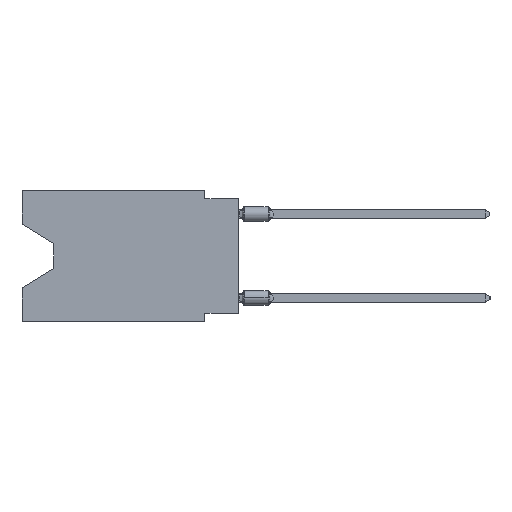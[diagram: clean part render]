
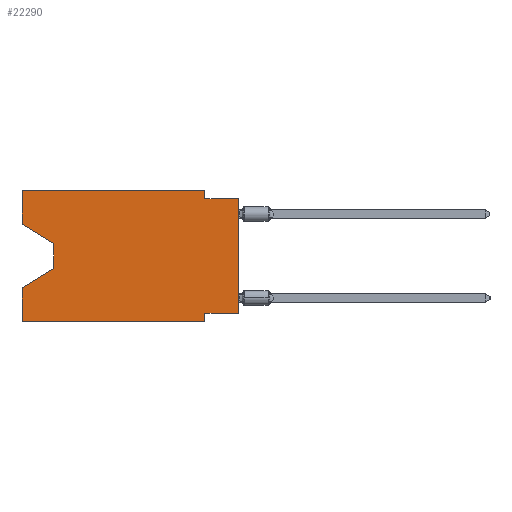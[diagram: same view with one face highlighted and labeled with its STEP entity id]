
A CAD part, left-side view. The second image highlights one B-rep face of the part: STEP entity #22290.
In plain terms, the highlighted planar face has unit normal (-1, 0, 0).
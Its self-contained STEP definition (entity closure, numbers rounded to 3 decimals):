
#914 = ORIENTED_EDGE ( 'NONE', *, *, #37291, .T. ) ;
#1246 = VECTOR ( 'NONE', #50071, 1000. ) ;
#2125 = FACE_OUTER_BOUND ( 'NONE', #40277, .T. ) ;
#2347 = LINE ( 'NONE', #66242, #57676 ) ;
#2634 = ORIENTED_EDGE ( 'NONE', *, *, #29283, .T. ) ;
#2832 = CARTESIAN_POINT ( 'NONE',  ( 0., 16.383, 0. ) ) ;
#3157 = CARTESIAN_POINT ( 'NONE',  ( 0., 0., -9.271 ) ) ;
#3553 = CARTESIAN_POINT ( 'NONE',  ( 0., 13.97, -5.893 ) ) ;
#3563 = ORIENTED_EDGE ( 'NONE', *, *, #9586, .F. ) ;
#4128 = VERTEX_POINT ( 'NONE', #50631 ) ;
#4748 = CARTESIAN_POINT ( 'NONE',  ( 0., 16.383, 0. ) ) ;
#4784 = ORIENTED_EDGE ( 'NONE', *, *, #48665, .F. ) ;
#5268 = LINE ( 'NONE', #67221, #38157 ) ;
#5447 = VERTEX_POINT ( 'NONE', #4748 ) ;
#6087 = CARTESIAN_POINT ( 'NONE',  ( 0., 2.54, 0. ) ) ;
#6131 = EDGE_CURVE ( 'NONE', #46796, #10814, #5268, .T. ) ;
#6180 = CARTESIAN_POINT ( 'NONE',  ( 0., 0., 0. ) ) ;
#6222 = VECTOR ( 'NONE', #42809, 1000. ) ;
#8156 = VERTEX_POINT ( 'NONE', #3553 ) ;
#9586 = EDGE_CURVE ( 'NONE', #55805, #35050, #18229, .T. ) ;
#9799 = EDGE_CURVE ( 'NONE', #63018, #8156, #32179, .T. ) ;
#10131 = ORIENTED_EDGE ( 'NONE', *, *, #9799, .T. ) ;
#10814 = VERTEX_POINT ( 'NONE', #50067 ) ;
#11669 = DIRECTION ( 'NONE',  ( 0., 0., 1. ) ) ;
#11736 = EDGE_CURVE ( 'NONE', #55805, #40909, #49175, .T. ) ;
#12637 = DIRECTION ( 'NONE',  ( 0., 0.855, -0.519 ) ) ;
#12690 = LINE ( 'NONE', #6180, #13925 ) ;
#12749 = VECTOR ( 'NONE', #59636, 1000. ) ;
#12761 = DIRECTION ( 'NONE',  ( 0., 0., -1. ) ) ;
#13824 = CARTESIAN_POINT ( 'NONE',  ( 0., 2.54, -9.906 ) ) ;
#13925 = VECTOR ( 'NONE', #11669, 1000. ) ;
#14439 = LINE ( 'NONE', #3157, #66631 ) ;
#14901 = DIRECTION ( 'NONE',  ( 0., 0., -1. ) ) ;
#15201 = DIRECTION ( 'NONE',  ( 0., -1., 0. ) ) ;
#16277 = VECTOR ( 'NONE', #25851, 1000. ) ;
#16648 = VERTEX_POINT ( 'NONE', #6087 ) ;
#17087 = CARTESIAN_POINT ( 'NONE',  ( 0., 16.383, 0. ) ) ;
#17767 = DIRECTION ( 'NONE',  ( 0., 0., 1. ) ) ;
#18229 = LINE ( 'NONE', #43891, #12749 ) ;
#18454 = ORIENTED_EDGE ( 'NONE', *, *, #25771, .F. ) ;
#18570 = DIRECTION ( 'NONE',  ( 0., 1., 0. ) ) ;
#21755 = LINE ( 'NONE', #53243, #16277 ) ;
#22000 = DIRECTION ( 'NONE',  ( 1., 0., 0. ) ) ;
#22219 = LINE ( 'NONE', #17087, #60879 ) ;
#22290 = ADVANCED_FACE ( 'NONE', ( #2125 ), #37730, .F. ) ;
#23151 = CARTESIAN_POINT ( 'NONE',  ( 0., 16.383, -9.906 ) ) ;
#25771 = EDGE_CURVE ( 'NONE', #4128, #40909, #51959, .T. ) ;
#25851 = DIRECTION ( 'NONE',  ( 0., -0.855, -0.519 ) ) ;
#26145 = ORIENTED_EDGE ( 'NONE', *, *, #6131, .F. ) ;
#26645 = VERTEX_POINT ( 'NONE', #52737 ) ;
#29283 = EDGE_CURVE ( 'NONE', #34158, #10814, #12690, .T. ) ;
#30718 = CARTESIAN_POINT ( 'NONE',  ( 0., 0., -9.271 ) ) ;
#32179 = LINE ( 'NONE', #47275, #6222 ) ;
#34158 = VERTEX_POINT ( 'NONE', #30718 ) ;
#34638 = LINE ( 'NONE', #2832, #1246 ) ;
#35050 = VERTEX_POINT ( 'NONE', #61635 ) ;
#36134 = CARTESIAN_POINT ( 'NONE',  ( 0., 16.383, -9.906 ) ) ;
#36195 = CARTESIAN_POINT ( 'NONE',  ( 0., 2.54, -9.906 ) ) ;
#37291 = EDGE_CURVE ( 'NONE', #26645, #63018, #21755, .T. ) ;
#37491 = ORIENTED_EDGE ( 'NONE', *, *, #47488, .T. ) ;
#37730 = PLANE ( 'NONE',  #50889 ) ;
#37990 = EDGE_CURVE ( 'NONE', #34158, #4128, #14439, .T. ) ;
#38084 = ORIENTED_EDGE ( 'NONE', *, *, #56380, .F. ) ;
#38157 = VECTOR ( 'NONE', #15201, 1000. ) ;
#39577 = DIRECTION ( 'NONE',  ( 0., -1., 0. ) ) ;
#40277 = EDGE_LOOP ( 'NONE', ( #914, #10131, #37491, #3563, #63450, #18454, #47755, #2634, #26145, #59065, #38084, #4784 ) ) ;
#40909 = VERTEX_POINT ( 'NONE', #13824 ) ;
#41551 = CARTESIAN_POINT ( 'NONE',  ( 0., 13.97, -4.013 ) ) ;
#41683 = DIRECTION ( 'NONE',  ( 0., 0., -1. ) ) ;
#42809 = DIRECTION ( 'NONE',  ( 0., 0., -1. ) ) ;
#43891 = CARTESIAN_POINT ( 'NONE',  ( 0., 16.383, 0. ) ) ;
#46796 = VERTEX_POINT ( 'NONE', #61364 ) ;
#47275 = CARTESIAN_POINT ( 'NONE',  ( 0., 13.97, -4.013 ) ) ;
#47488 = EDGE_CURVE ( 'NONE', #8156, #35050, #2347, .T. ) ;
#47755 = ORIENTED_EDGE ( 'NONE', *, *, #37990, .F. ) ;
#48665 = EDGE_CURVE ( 'NONE', #26645, #5447, #22219, .T. ) ;
#48683 = CARTESIAN_POINT ( 'NONE',  ( 0., 16.383, 0. ) ) ;
#49175 = LINE ( 'NONE', #23151, #55588 ) ;
#49393 = EDGE_CURVE ( 'NONE', #16648, #46796, #62118, .T. ) ;
#50067 = CARTESIAN_POINT ( 'NONE',  ( 0., 0., -0.635 ) ) ;
#50071 = DIRECTION ( 'NONE',  ( 0., -1., 0. ) ) ;
#50631 = CARTESIAN_POINT ( 'NONE',  ( 0., 2.54, -9.271 ) ) ;
#50889 = AXIS2_PLACEMENT_3D ( 'NONE', #48683, #22000, #12761 ) ;
#51959 = LINE ( 'NONE', #36195, #65058 ) ;
#52737 = CARTESIAN_POINT ( 'NONE',  ( 0., 16.383, -2.546 ) ) ;
#53243 = CARTESIAN_POINT ( 'NONE',  ( 0., 16.383, -2.546 ) ) ;
#55588 = VECTOR ( 'NONE', #39577, 1000. ) ;
#55805 = VERTEX_POINT ( 'NONE', #36134 ) ;
#56380 = EDGE_CURVE ( 'NONE', #5447, #16648, #34638, .T. ) ;
#57676 = VECTOR ( 'NONE', #12637, 1000. ) ;
#59065 = ORIENTED_EDGE ( 'NONE', *, *, #49393, .F. ) ;
#59636 = DIRECTION ( 'NONE',  ( 0., 0., 1. ) ) ;
#60879 = VECTOR ( 'NONE', #17767, 1000. ) ;
#61364 = CARTESIAN_POINT ( 'NONE',  ( 0., 2.54, -0.635 ) ) ;
#61635 = CARTESIAN_POINT ( 'NONE',  ( 0., 16.383, -7.36 ) ) ;
#61780 = CARTESIAN_POINT ( 'NONE',  ( 0., 2.54, 0. ) ) ;
#61997 = VECTOR ( 'NONE', #14901, 1000. ) ;
#62118 = LINE ( 'NONE', #61780, #61997 ) ;
#63018 = VERTEX_POINT ( 'NONE', #41551 ) ;
#63450 = ORIENTED_EDGE ( 'NONE', *, *, #11736, .T. ) ;
#65058 = VECTOR ( 'NONE', #41683, 1000. ) ;
#66242 = CARTESIAN_POINT ( 'NONE',  ( 0., 13.97, -5.893 ) ) ;
#66631 = VECTOR ( 'NONE', #18570, 1000. ) ;
#67221 = CARTESIAN_POINT ( 'NONE',  ( 0., 0., -0.635 ) ) ;
